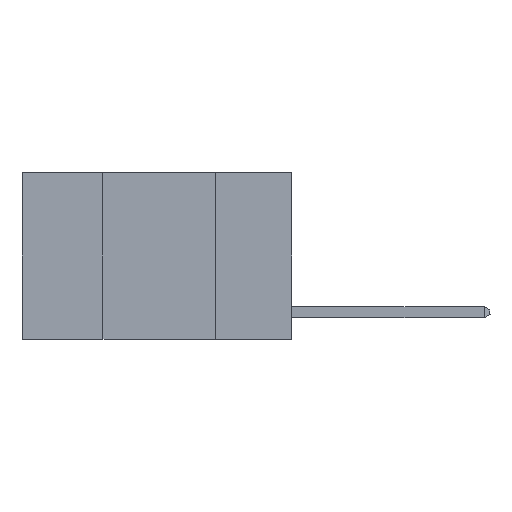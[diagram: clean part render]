
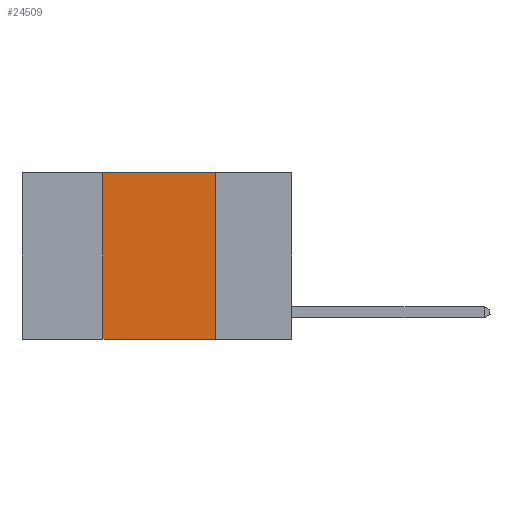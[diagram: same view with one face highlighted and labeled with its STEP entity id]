
A CAD part, left-side view. The second image highlights one B-rep face of the part: STEP entity #24509.
In plain terms, the highlighted planar face has unit normal (-1, 0, 0).
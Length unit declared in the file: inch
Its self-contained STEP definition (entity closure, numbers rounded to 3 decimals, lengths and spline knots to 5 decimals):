
#1038 = VERTEX_POINT ( 'NONE', #17295 ) ;
#1780 = ORIENTED_EDGE ( 'NONE', *, *, #11748, .F. ) ;
#3920 = VECTOR ( 'NONE', #12558, 39.37008 ) ;
#4179 = VECTOR ( 'NONE', #5812, 39.37008 ) ;
#5310 = ORIENTED_EDGE ( 'NONE', *, *, #21280, .F. ) ;
#5528 = CARTESIAN_POINT ( 'NONE',  ( 0., 0.42, -0.37 ) ) ;
#5591 = AXIS2_PLACEMENT_3D ( 'NONE', #15178, #23845, #19848 ) ;
#5812 = DIRECTION ( 'NONE',  ( 0., -1., 0. ) ) ;
#7575 = CARTESIAN_POINT ( 'NONE',  ( 0., 0.42, 0. ) ) ;
#7905 = EDGE_CURVE ( 'NONE', #1038, #26630, #16061, .T. ) ;
#8148 = ORIENTED_EDGE ( 'NONE', *, *, #22779, .T. ) ;
#8632 = FACE_OUTER_BOUND ( 'NONE', #23278, .T. ) ;
#9354 = CARTESIAN_POINT ( 'NONE',  ( 0., 0.17, 0. ) ) ;
#11748 = EDGE_CURVE ( 'NONE', #24136, #25198, #28043, .T. ) ;
#12558 = DIRECTION ( 'NONE',  ( 0., 0., 1. ) ) ;
#12822 = VECTOR ( 'NONE', #23753, 39.37008 ) ;
#13799 = ORIENTED_EDGE ( 'NONE', *, *, #7905, .F. ) ;
#15178 = CARTESIAN_POINT ( 'NONE',  ( 0., 0.6, 0. ) ) ;
#15229 = CARTESIAN_POINT ( 'NONE',  ( 0., 0.42, 0. ) ) ;
#15464 = PLANE ( 'NONE',  #5591 ) ;
#15774 = DIRECTION ( 'NONE',  ( 0., 0., -1. ) ) ;
#16061 = LINE ( 'NONE', #9354, #25079 ) ;
#17295 = CARTESIAN_POINT ( 'NONE',  ( 0., 0.17, 0. ) ) ;
#17315 = CARTESIAN_POINT ( 'NONE',  ( 0., 0.6, 0. ) ) ;
#19616 = CARTESIAN_POINT ( 'NONE',  ( 0., 0.6, -0.37 ) ) ;
#19848 = DIRECTION ( 'NONE',  ( 0., 0., -1. ) ) ;
#21280 = EDGE_CURVE ( 'NONE', #25198, #1038, #27873, .T. ) ;
#22779 = EDGE_CURVE ( 'NONE', #24136, #26630, #25894, .T. ) ;
#23278 = EDGE_LOOP ( 'NONE', ( #13799, #5310, #1780, #8148 ) ) ;
#23753 = DIRECTION ( 'NONE',  ( 0., -1., 0. ) ) ;
#23845 = DIRECTION ( 'NONE',  ( 1., 0., 0. ) ) ;
#24136 = VERTEX_POINT ( 'NONE', #5528 ) ;
#24509 = ADVANCED_FACE ( 'NONE', ( #8632 ), #15464, .F. ) ;
#25079 = VECTOR ( 'NONE', #15774, 39.37008 ) ;
#25198 = VERTEX_POINT ( 'NONE', #7575 ) ;
#25894 = LINE ( 'NONE', #19616, #12822 ) ;
#26599 = CARTESIAN_POINT ( 'NONE',  ( 0., 0.17, -0.37 ) ) ;
#26630 = VERTEX_POINT ( 'NONE', #26599 ) ;
#27873 = LINE ( 'NONE', #17315, #4179 ) ;
#28043 = LINE ( 'NONE', #15229, #3920 ) ;
